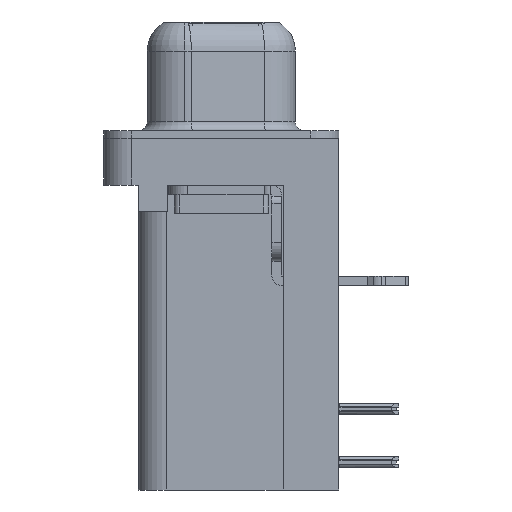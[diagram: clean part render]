
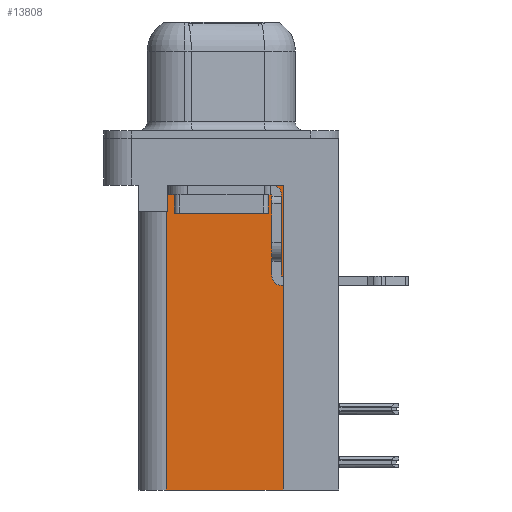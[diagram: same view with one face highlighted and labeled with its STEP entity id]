
A CAD part, left-side view. The second image highlights one B-rep face of the part: STEP entity #13808.
In plain terms, the highlighted planar face has unit normal (-1, 0, 0).
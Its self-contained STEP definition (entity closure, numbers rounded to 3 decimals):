
#651 = CARTESIAN_POINT ( 'NONE',  ( 3.7, -3.295, -18.76 ) ) ;
#1824 = PLANE ( 'NONE',  #23886 ) ;
#2368 = LINE ( 'NONE', #25937, #2398 ) ;
#2398 = VECTOR ( 'NONE', #21736, 1000. ) ;
#2971 = CARTESIAN_POINT ( 'NONE',  ( 3.7, -3.295, -18.76 ) ) ;
#3213 = VECTOR ( 'NONE', #10435, 1000. ) ;
#3297 = LINE ( 'NONE', #5592, #3213 ) ;
#3865 = VERTEX_POINT ( 'NONE', #14318 ) ;
#4366 = ORIENTED_EDGE ( 'NONE', *, *, #19045, .T. ) ;
#4885 = ORIENTED_EDGE ( 'NONE', *, *, #20587, .T. ) ;
#5171 = ORIENTED_EDGE ( 'NONE', *, *, #27372, .T. ) ;
#5592 = CARTESIAN_POINT ( 'NONE',  ( 3.7, 2.925, -18.76 ) ) ;
#6307 = VERTEX_POINT ( 'NONE', #12544 ) ;
#6511 = ORIENTED_EDGE ( 'NONE', *, *, #16803, .T. ) ;
#7297 = CARTESIAN_POINT ( 'NONE',  ( 3.7, -3.295, -2.5 ) ) ;
#7978 = DIRECTION ( 'NONE',  ( 0., 1., 0. ) ) ;
#8960 = DIRECTION ( 'NONE',  ( 1., 0., 0. ) ) ;
#10089 = VERTEX_POINT ( 'NONE', #651 ) ;
#10435 = DIRECTION ( 'NONE',  ( 0., 0., 1. ) ) ;
#10989 = CARTESIAN_POINT ( 'NONE',  ( 3.7, 2.895, -3.9 ) ) ;
#12544 = CARTESIAN_POINT ( 'NONE',  ( 3.7, -3.295, -2.5 ) ) ;
#13617 = ORIENTED_EDGE ( 'NONE', *, *, #26080, .F. ) ;
#13620 = CARTESIAN_POINT ( 'NONE',  ( 3.7, -3.295, -18.76 ) ) ;
#13808 = ADVANCED_FACE ( 'NONE', ( #18419 ), #1824, .F. ) ;
#13876 = VERTEX_POINT ( 'NONE', #13939 ) ;
#13939 = CARTESIAN_POINT ( 'NONE',  ( 3.7, 2.925, -18.76 ) ) ;
#14318 = CARTESIAN_POINT ( 'NONE',  ( 3.7, 2.925, -3.9 ) ) ;
#14818 = DIRECTION ( 'NONE',  ( 0., 1., 0. ) ) ;
#15261 = CARTESIAN_POINT ( 'NONE',  ( 3.7, -3.295, -18.76 ) ) ;
#16803 = EDGE_CURVE ( 'NONE', #6307, #27892, #18273, .T. ) ;
#17120 = ORIENTED_EDGE ( 'NONE', *, *, #27214, .F. ) ;
#17683 = DIRECTION ( 'NONE',  ( 0., 0., 1. ) ) ;
#18027 = VERTEX_POINT ( 'NONE', #10989 ) ;
#18216 = VECTOR ( 'NONE', #14818, 1000. ) ;
#18273 = LINE ( 'NONE', #7297, #18216 ) ;
#18419 = FACE_OUTER_BOUND ( 'NONE', #22462, .T. ) ;
#19045 = EDGE_CURVE ( 'NONE', #27892, #18027, #2368, .T. ) ;
#19623 = DIRECTION ( 'NONE',  ( 0., 1., 0. ) ) ;
#20587 = EDGE_CURVE ( 'NONE', #18027, #3865, #23899, .T. ) ;
#21402 = VECTOR ( 'NONE', #17683, 1000. ) ;
#21736 = DIRECTION ( 'NONE',  ( 0., 0., -1. ) ) ;
#21785 = LINE ( 'NONE', #15261, #21402 ) ;
#22006 = CARTESIAN_POINT ( 'NONE',  ( 3.7, 0., -3.9 ) ) ;
#22462 = EDGE_LOOP ( 'NONE', ( #6511, #4366, #4885, #13617, #17120, #5171 ) ) ;
#22799 = LINE ( 'NONE', #2971, #23107 ) ;
#23107 = VECTOR ( 'NONE', #19623, 1000. ) ;
#23871 = VECTOR ( 'NONE', #7978, 1000. ) ;
#23886 = AXIS2_PLACEMENT_3D ( 'NONE', #13620, #8960, #24969 ) ;
#23899 = LINE ( 'NONE', #22006, #23871 ) ;
#24969 = DIRECTION ( 'NONE',  ( 0., 1., 0. ) ) ;
#25937 = CARTESIAN_POINT ( 'NONE',  ( 3.7, 2.895, -3.9 ) ) ;
#26080 = EDGE_CURVE ( 'NONE', #13876, #3865, #3297, .T. ) ;
#27214 = EDGE_CURVE ( 'NONE', #10089, #13876, #22799, .T. ) ;
#27372 = EDGE_CURVE ( 'NONE', #10089, #6307, #21785, .T. ) ;
#27892 = VERTEX_POINT ( 'NONE', #28133 ) ;
#28133 = CARTESIAN_POINT ( 'NONE',  ( 3.7, 2.895, -2.5 ) ) ;
